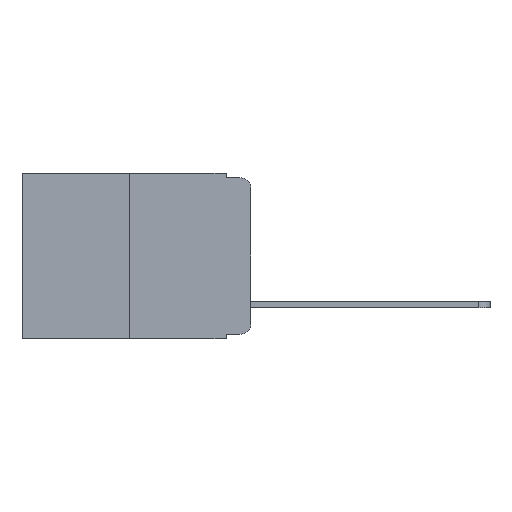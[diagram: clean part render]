
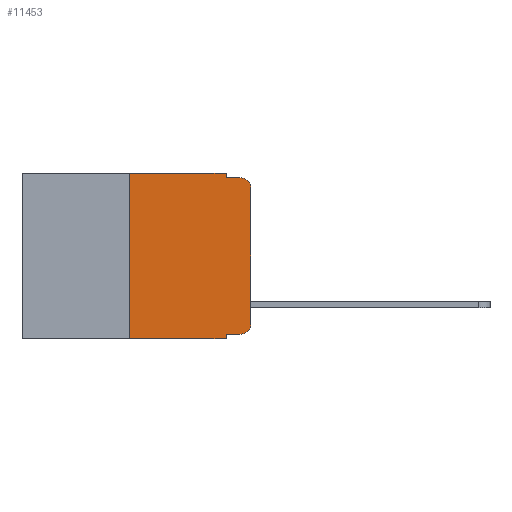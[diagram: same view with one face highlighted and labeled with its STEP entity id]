
A CAD part, left-side view. The second image highlights one B-rep face of the part: STEP entity #11453.
In plain terms, the highlighted planar face has unit normal (-1, 0, 0).
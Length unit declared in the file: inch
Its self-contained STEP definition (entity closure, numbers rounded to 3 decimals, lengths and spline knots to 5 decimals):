
#273 = EDGE_CURVE ( 'NONE', #3489, #1475, #7385, .T. ) ;
#636 = CARTESIAN_POINT ( 'NONE',  ( 0., 0.051, -0.343 ) ) ;
#1135 = VERTEX_POINT ( 'NONE', #10487 ) ;
#1292 = LINE ( 'NONE', #10028, #5382 ) ;
#1475 = VERTEX_POINT ( 'NONE', #5076 ) ;
#1688 = VERTEX_POINT ( 'NONE', #13532 ) ;
#1951 = VERTEX_POINT ( 'NONE', #8163 ) ;
#2338 = EDGE_CURVE ( 'NONE', #1951, #4929, #4281, .T. ) ;
#2658 = DIRECTION ( 'NONE',  ( 0., 0., -1. ) ) ;
#2795 = CARTESIAN_POINT ( 'NONE',  ( 0., 0., -0.313 ) ) ;
#2894 = EDGE_LOOP ( 'NONE', ( #14317, #13937, #8655, #6673, #3108, #13199, #13611, #3302, #3613, #2953 ) ) ;
#2953 = ORIENTED_EDGE ( 'NONE', *, *, #8310, .T. ) ;
#3108 = ORIENTED_EDGE ( 'NONE', *, *, #273, .F. ) ;
#3302 = ORIENTED_EDGE ( 'NONE', *, *, #12440, .F. ) ;
#3489 = VERTEX_POINT ( 'NONE', #12057 ) ;
#3504 = DIRECTION ( 'NONE',  ( 0., 0., -1. ) ) ;
#3613 = ORIENTED_EDGE ( 'NONE', *, *, #11719, .T. ) ;
#3621 = DIRECTION ( 'NONE',  ( 0., -1., 0. ) ) ;
#3651 = DIRECTION ( 'NONE',  ( 1., 0., 0. ) ) ;
#3927 = DIRECTION ( 'NONE',  ( 0., 0., 1. ) ) ;
#4281 = LINE ( 'NONE', #14018, #4625 ) ;
#4321 = LINE ( 'NONE', #6345, #5217 ) ;
#4509 = EDGE_CURVE ( 'NONE', #8243, #4929, #9459, .T. ) ;
#4625 = VECTOR ( 'NONE', #13026, 39.37008 ) ;
#4929 = VERTEX_POINT ( 'NONE', #7422 ) ;
#5076 = CARTESIAN_POINT ( 'NONE',  ( 0., 0.051, 0. ) ) ;
#5217 = VECTOR ( 'NONE', #14381, 39.37008 ) ;
#5245 = VECTOR ( 'NONE', #8890, 39.37008 ) ;
#5252 = VERTEX_POINT ( 'NONE', #636 ) ;
#5277 = AXIS2_PLACEMENT_3D ( 'NONE', #6012, #3651, #2658 ) ;
#5382 = VECTOR ( 'NONE', #3927, 39.37008 ) ;
#6012 = CARTESIAN_POINT ( 'NONE',  ( 0., 0.473, 0. ) ) ;
#6345 = CARTESIAN_POINT ( 'NONE',  ( 0., 0.473, -0.343 ) ) ;
#6499 = LINE ( 'NONE', #8792, #5245 ) ;
#6557 = AXIS2_PLACEMENT_3D ( 'NONE', #13475, #10170, #6806 ) ;
#6673 = ORIENTED_EDGE ( 'NONE', *, *, #8816, .F. ) ;
#6806 = DIRECTION ( 'NONE',  ( 0., 0., -1. ) ) ;
#6831 = CARTESIAN_POINT ( 'NONE',  ( 0., 0., -0.03 ) ) ;
#7031 = EDGE_CURVE ( 'NONE', #11941, #3489, #6499, .T. ) ;
#7229 = VECTOR ( 'NONE', #3621, 39.37008 ) ;
#7385 = LINE ( 'NONE', #13221, #13418 ) ;
#7422 = CARTESIAN_POINT ( 'NONE',  ( 0., 0.02, -0.01 ) ) ;
#7470 = AXIS2_PLACEMENT_3D ( 'NONE', #12076, #12959, #13003 ) ;
#8025 = VERTEX_POINT ( 'NONE', #2795 ) ;
#8163 = CARTESIAN_POINT ( 'NONE',  ( 0., 0.051, -0.01 ) ) ;
#8240 = CIRCLE ( 'NONE', #7470, 0.02 ) ;
#8243 = VERTEX_POINT ( 'NONE', #6831 ) ;
#8310 = EDGE_CURVE ( 'NONE', #1688, #8025, #8240, .T. ) ;
#8655 = ORIENTED_EDGE ( 'NONE', *, *, #2338, .F. ) ;
#8792 = CARTESIAN_POINT ( 'NONE',  ( 0., 0.25, 0. ) ) ;
#8816 = EDGE_CURVE ( 'NONE', #1475, #1951, #12662, .T. ) ;
#8890 = DIRECTION ( 'NONE',  ( 0., 0., 1. ) ) ;
#9459 = CIRCLE ( 'NONE', #6557, 0.02 ) ;
#10028 = CARTESIAN_POINT ( 'NONE',  ( 0., 0., 0. ) ) ;
#10170 = DIRECTION ( 'NONE',  ( -1., 0., 0. ) ) ;
#10487 = CARTESIAN_POINT ( 'NONE',  ( 0., 0.051, -0.333 ) ) ;
#10570 = PLANE ( 'NONE',  #5277 ) ;
#10599 = LINE ( 'NONE', #13870, #12701 ) ;
#11453 = ADVANCED_FACE ( 'NONE', ( #14172 ), #10570, .F. ) ;
#11719 = EDGE_CURVE ( 'NONE', #1135, #1688, #14505, .T. ) ;
#11941 = VERTEX_POINT ( 'NONE', #13097 ) ;
#12057 = CARTESIAN_POINT ( 'NONE',  ( 0., 0.25, 0. ) ) ;
#12076 = CARTESIAN_POINT ( 'NONE',  ( 0., 0.02, -0.313 ) ) ;
#12217 = DIRECTION ( 'NONE',  ( 0., -1., 0. ) ) ;
#12440 = EDGE_CURVE ( 'NONE', #1135, #5252, #10599, .T. ) ;
#12586 = EDGE_CURVE ( 'NONE', #11941, #5252, #4321, .T. ) ;
#12662 = LINE ( 'NONE', #12865, #14268 ) ;
#12701 = VECTOR ( 'NONE', #3504, 39.37008 ) ;
#12811 = DIRECTION ( 'NONE',  ( 0., 0., -1. ) ) ;
#12865 = CARTESIAN_POINT ( 'NONE',  ( 0., 0.051, 0. ) ) ;
#12909 = EDGE_CURVE ( 'NONE', #8025, #8243, #1292, .T. ) ;
#12959 = DIRECTION ( 'NONE',  ( -1., 0., 0. ) ) ;
#13003 = DIRECTION ( 'NONE',  ( 0., 0., -1. ) ) ;
#13026 = DIRECTION ( 'NONE',  ( 0., -1., 0. ) ) ;
#13097 = CARTESIAN_POINT ( 'NONE',  ( 0., 0.25, -0.343 ) ) ;
#13199 = ORIENTED_EDGE ( 'NONE', *, *, #7031, .F. ) ;
#13221 = CARTESIAN_POINT ( 'NONE',  ( 0., 0.473, 0. ) ) ;
#13418 = VECTOR ( 'NONE', #12217, 39.37008 ) ;
#13475 = CARTESIAN_POINT ( 'NONE',  ( 0., 0.02, -0.03 ) ) ;
#13532 = CARTESIAN_POINT ( 'NONE',  ( 0., 0.02, -0.333 ) ) ;
#13611 = ORIENTED_EDGE ( 'NONE', *, *, #12586, .T. ) ;
#13870 = CARTESIAN_POINT ( 'NONE',  ( 0., 0.051, 0. ) ) ;
#13937 = ORIENTED_EDGE ( 'NONE', *, *, #4509, .T. ) ;
#14018 = CARTESIAN_POINT ( 'NONE',  ( 0., 0.051, -0.01 ) ) ;
#14035 = CARTESIAN_POINT ( 'NONE',  ( 0., 0.051, -0.333 ) ) ;
#14172 = FACE_OUTER_BOUND ( 'NONE', #2894, .T. ) ;
#14268 = VECTOR ( 'NONE', #12811, 39.37008 ) ;
#14317 = ORIENTED_EDGE ( 'NONE', *, *, #12909, .T. ) ;
#14381 = DIRECTION ( 'NONE',  ( 0., -1., 0. ) ) ;
#14505 = LINE ( 'NONE', #14035, #7229 ) ;
